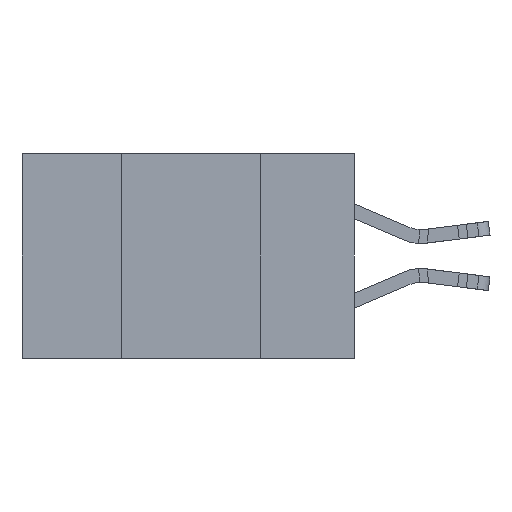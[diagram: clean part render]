
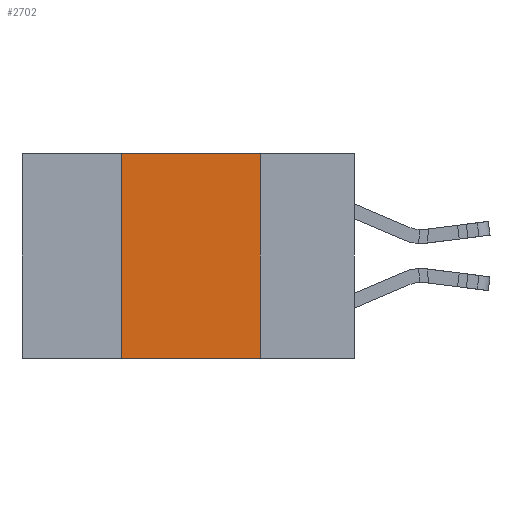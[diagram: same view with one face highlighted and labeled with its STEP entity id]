
A CAD part, left-side view. The second image highlights one B-rep face of the part: STEP entity #2702.
In plain terms, the highlighted planar face has unit normal (-1, 0, 0).
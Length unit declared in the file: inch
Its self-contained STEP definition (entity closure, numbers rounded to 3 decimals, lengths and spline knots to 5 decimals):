
#1750 = CARTESIAN_POINT ( 'NONE',  ( 0., 0.17, -0.37 ) ) ;
#2101 = CARTESIAN_POINT ( 'NONE',  ( 0., 0.42, 0. ) ) ;
#2133 = DIRECTION ( 'NONE',  ( 0., 0., -1. ) ) ;
#2702 = ADVANCED_FACE ( 'NONE', ( #17218 ), #31045, .F. ) ;
#2774 = VERTEX_POINT ( 'NONE', #1750 ) ;
#4145 = VECTOR ( 'NONE', #9341, 39.37008 ) ;
#4770 = CARTESIAN_POINT ( 'NONE',  ( 0., 0.17, 0. ) ) ;
#5699 = EDGE_CURVE ( 'NONE', #11158, #2774, #26825, .T. ) ;
#6288 = VERTEX_POINT ( 'NONE', #2101 ) ;
#6862 = LINE ( 'NONE', #11604, #20447 ) ;
#7684 = CARTESIAN_POINT ( 'NONE',  ( 0., 0.6, -0.37 ) ) ;
#8248 = DIRECTION ( 'NONE',  ( 0., -1., 0. ) ) ;
#8446 = EDGE_CURVE ( 'NONE', #6288, #21222, #25379, .T. ) ;
#9341 = DIRECTION ( 'NONE',  ( 0., 0., -1. ) ) ;
#11158 = VERTEX_POINT ( 'NONE', #26676 ) ;
#11604 = CARTESIAN_POINT ( 'NONE',  ( 0., 0.42, 0. ) ) ;
#13470 = VECTOR ( 'NONE', #18473, 39.37008 ) ;
#14330 = DIRECTION ( 'NONE',  ( 0., 0., 1. ) ) ;
#17218 = FACE_OUTER_BOUND ( 'NONE', #26333, .T. ) ;
#18473 = DIRECTION ( 'NONE',  ( 0., -1., 0. ) ) ;
#18602 = LINE ( 'NONE', #20096, #4145 ) ;
#19650 = ORIENTED_EDGE ( 'NONE', *, *, #8446, .F. ) ;
#20096 = CARTESIAN_POINT ( 'NONE',  ( 0., 0.17, 0. ) ) ;
#20447 = VECTOR ( 'NONE', #14330, 39.37008 ) ;
#21222 = VERTEX_POINT ( 'NONE', #4770 ) ;
#22957 = ORIENTED_EDGE ( 'NONE', *, *, #28076, .F. ) ;
#23967 = ORIENTED_EDGE ( 'NONE', *, *, #5699, .T. ) ;
#25379 = LINE ( 'NONE', #27181, #31567 ) ;
#26093 = DIRECTION ( 'NONE',  ( 1., 0., 0. ) ) ;
#26284 = EDGE_CURVE ( 'NONE', #11158, #6288, #6862, .T. ) ;
#26333 = EDGE_LOOP ( 'NONE', ( #22957, #19650, #27807, #23967 ) ) ;
#26676 = CARTESIAN_POINT ( 'NONE',  ( 0., 0.42, -0.37 ) ) ;
#26825 = LINE ( 'NONE', #7684, #13470 ) ;
#27181 = CARTESIAN_POINT ( 'NONE',  ( 0., 0.6, 0. ) ) ;
#27807 = ORIENTED_EDGE ( 'NONE', *, *, #26284, .F. ) ;
#28076 = EDGE_CURVE ( 'NONE', #21222, #2774, #18602, .T. ) ;
#28160 = AXIS2_PLACEMENT_3D ( 'NONE', #34453, #26093, #2133 ) ;
#31045 = PLANE ( 'NONE',  #28160 ) ;
#31567 = VECTOR ( 'NONE', #8248, 39.37008 ) ;
#34453 = CARTESIAN_POINT ( 'NONE',  ( 0., 0.6, 0. ) ) ;
